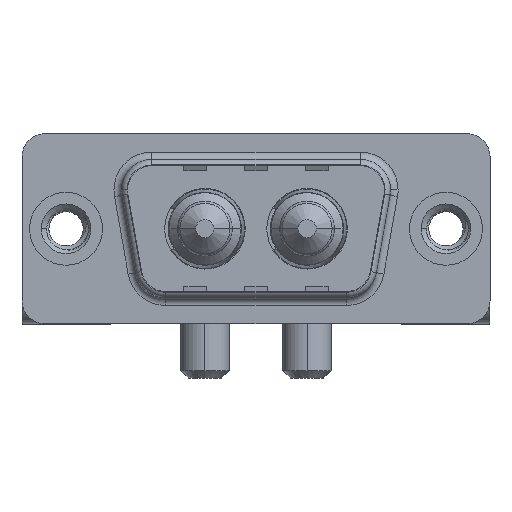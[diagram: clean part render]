
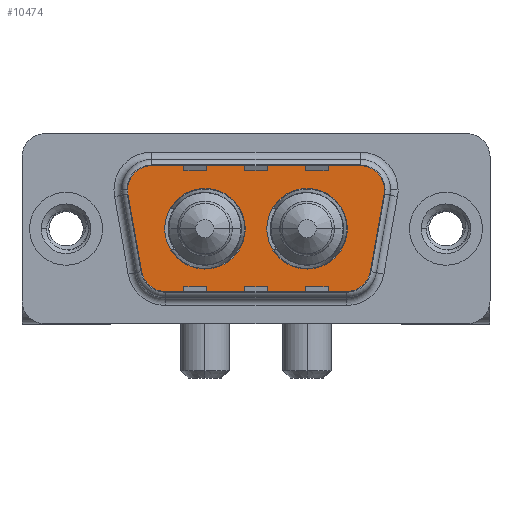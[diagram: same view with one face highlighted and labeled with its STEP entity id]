
A CAD part, top view. The second image highlights one B-rep face of the part: STEP entity #10474.
In plain terms, the highlighted planar face has unit normal (0, 0, 1).
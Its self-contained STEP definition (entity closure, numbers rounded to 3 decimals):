
#266 = CARTESIAN_POINT ( 'NONE',  ( 18.51, 0., 0. ) ) ;
#269 = CARTESIAN_POINT ( 'NONE',  ( 11.79, 0., 0. ) ) ;
#540 = EDGE_CURVE ( 'NONE', #4864, #10879, #11350, .T. ) ;
#550 = DIRECTION ( 'NONE',  ( 1., 0., 0. ) ) ;
#555 = ORIENTED_EDGE ( 'NONE', *, *, #4746, .T. ) ;
#648 = CARTESIAN_POINT ( 'NONE',  ( 5.436, 4.9, 0. ) ) ;
#845 = LINE ( 'NONE', #12289, #9375 ) ;
#884 = CARTESIAN_POINT ( 'NONE',  ( 6.459, -4.9, 0. ) ) ;
#1030 = FACE_OUTER_BOUND ( 'NONE', #4273, .T. ) ;
#1350 = VERTEX_POINT ( 'NONE', #11225 ) ;
#1353 = CARTESIAN_POINT ( 'NONE',  ( 18.541, -4.9, 0. ) ) ;
#1484 = VERTEX_POINT ( 'NONE', #8510 ) ;
#1983 = CARTESIAN_POINT ( 'NONE',  ( 6.459, -4.9, 0. ) ) ;
#2036 = CARTESIAN_POINT ( 'NONE',  ( 9.14, 0., 0. ) ) ;
#2043 = DIRECTION ( 'NONE',  ( 1., 0., 0. ) ) ;
#2102 = CARTESIAN_POINT ( 'NONE',  ( 18.541, -2.9, 0. ) ) ;
#2132 = EDGE_LOOP ( 'NONE', ( #4965, #3068 ) ) ;
#2228 = AXIS2_PLACEMENT_3D ( 'NONE', #5173, #6250, #6369 ) ;
#2273 = VERTEX_POINT ( 'NONE', #12430 ) ;
#2414 = VECTOR ( 'NONE', #12393, 1000. ) ;
#2449 = CARTESIAN_POINT ( 'NONE',  ( 5.436, 2.9, 0. ) ) ;
#2561 = LINE ( 'NONE', #6303, #6663 ) ;
#2609 = EDGE_CURVE ( 'NONE', #2273, #1484, #2561, .T. ) ;
#2627 = DIRECTION ( 'NONE',  ( 0.174, 0.985, 0. ) ) ;
#2643 = DIRECTION ( 'NONE',  ( 1., 0., 0. ) ) ;
#2693 = AXIS2_PLACEMENT_3D ( 'NONE', #9643, #8895, #9904 ) ;
#2695 = EDGE_CURVE ( 'NONE', #10616, #7680, #3641, .T. ) ;
#2728 = LINE ( 'NONE', #884, #2414 ) ;
#2748 = CARTESIAN_POINT ( 'NONE',  ( 15.86, 0., 0. ) ) ;
#2749 = VERTEX_POINT ( 'NONE', #269 ) ;
#2853 = AXIS2_PLACEMENT_3D ( 'NONE', #8465, #7459, #2643 ) ;
#2982 = ORIENTED_EDGE ( 'NONE', *, *, #3507, .F. ) ;
#2987 = DIRECTION ( 'NONE',  ( 0., 0., 1. ) ) ;
#3068 = ORIENTED_EDGE ( 'NONE', *, *, #9270, .F. ) ;
#3157 = AXIS2_PLACEMENT_3D ( 'NONE', #3383, #8386, #9260 ) ;
#3383 = CARTESIAN_POINT ( 'NONE',  ( 9.14, 0., 0. ) ) ;
#3507 = EDGE_CURVE ( 'NONE', #7680, #10616, #8321, .T. ) ;
#3641 = CIRCLE ( 'NONE', #8900, 2.65 ) ;
#3731 = CARTESIAN_POINT ( 'NONE',  ( 3.466, 2.553, 0. ) ) ;
#4209 = ORIENTED_EDGE ( 'NONE', *, *, #4969, .T. ) ;
#4273 = EDGE_LOOP ( 'NONE', ( #555, #5560, #10029, #4429, #10700, #5777, #8716, #11575, #4209 ) ) ;
#4429 = ORIENTED_EDGE ( 'NONE', *, *, #5820, .T. ) ;
#4691 = EDGE_CURVE ( 'NONE', #1484, #1350, #5625, .T. ) ;
#4746 = EDGE_CURVE ( 'NONE', #7253, #2273, #5834, .T. ) ;
#4842 = CARTESIAN_POINT ( 'NONE',  ( 6.49, 0., 0. ) ) ;
#4851 = EDGE_LOOP ( 'NONE', ( #5051, #2982 ) ) ;
#4864 = VERTEX_POINT ( 'NONE', #648 ) ;
#4965 = ORIENTED_EDGE ( 'NONE', *, *, #6888, .F. ) ;
#4969 = EDGE_CURVE ( 'NONE', #12478, #7253, #2728, .T. ) ;
#5015 = DIRECTION ( 'NONE',  ( -1., 0., 0. ) ) ;
#5051 = ORIENTED_EDGE ( 'NONE', *, *, #2695, .F. ) ;
#5173 = CARTESIAN_POINT ( 'NONE',  ( 19.564, 2.9, 0. ) ) ;
#5437 = AXIS2_PLACEMENT_3D ( 'NONE', #2102, #11718, #9818 ) ;
#5560 = ORIENTED_EDGE ( 'NONE', *, *, #2609, .T. ) ;
#5625 = CIRCLE ( 'NONE', #8866, 2. ) ;
#5742 = AXIS2_PLACEMENT_3D ( 'NONE', #7564, #2987, #2043 ) ;
#5777 = ORIENTED_EDGE ( 'NONE', *, *, #540, .T. ) ;
#5820 = EDGE_CURVE ( 'NONE', #1350, #9046, #8099, .T. ) ;
#5834 = CIRCLE ( 'NONE', #5437, 2. ) ;
#5887 = CARTESIAN_POINT ( 'NONE',  ( 5.436, 4.9, 0. ) ) ;
#6202 = VERTEX_POINT ( 'NONE', #10656 ) ;
#6218 = VERTEX_POINT ( 'NONE', #4842 ) ;
#6250 = DIRECTION ( 'NONE',  ( 0., 0., 1. ) ) ;
#6303 = CARTESIAN_POINT ( 'NONE',  ( 21.534, 2.553, 0. ) ) ;
#6369 = DIRECTION ( 'NONE',  ( -1., 0., 0. ) ) ;
#6539 = DIRECTION ( 'NONE',  ( 0., 0., 1. ) ) ;
#6663 = VECTOR ( 'NONE', #2627, 1000. ) ;
#6888 = EDGE_CURVE ( 'NONE', #2749, #6218, #10901, .T. ) ;
#6980 = DIRECTION ( 'NONE',  ( 0., 0., 1. ) ) ;
#7253 = VERTEX_POINT ( 'NONE', #1353 ) ;
#7459 = DIRECTION ( 'NONE',  ( 0., 0., 1. ) ) ;
#7564 = CARTESIAN_POINT ( 'NONE',  ( 18.541, -2.9, 0. ) ) ;
#7680 = VERTEX_POINT ( 'NONE', #10129 ) ;
#7810 = FACE_BOUND ( 'NONE', #2132, .T. ) ;
#7817 = CIRCLE ( 'NONE', #3157, 2.65 ) ;
#7994 = CARTESIAN_POINT ( 'NONE',  ( 19.564, 2.9, 0. ) ) ;
#8099 = CIRCLE ( 'NONE', #2228, 2. ) ;
#8321 = CIRCLE ( 'NONE', #2853, 2.65 ) ;
#8386 = DIRECTION ( 'NONE',  ( 0., 0., 1. ) ) ;
#8465 = CARTESIAN_POINT ( 'NONE',  ( 15.86, 0., 0. ) ) ;
#8510 = CARTESIAN_POINT ( 'NONE',  ( 21.534, 2.553, 0. ) ) ;
#8563 = DIRECTION ( 'NONE',  ( 0., 0., 1. ) ) ;
#8716 = ORIENTED_EDGE ( 'NONE', *, *, #12156, .T. ) ;
#8738 = LINE ( 'NONE', #5887, #8808 ) ;
#8802 = DIRECTION ( 'NONE',  ( 0.174, -0.985, 0. ) ) ;
#8808 = VECTOR ( 'NONE', #11516, 1000. ) ;
#8863 = EDGE_CURVE ( 'NONE', #9046, #4864, #8738, .T. ) ;
#8866 = AXIS2_PLACEMENT_3D ( 'NONE', #7994, #6980, #5015 ) ;
#8895 = DIRECTION ( 'NONE',  ( 0., 0., 1. ) ) ;
#8900 = AXIS2_PLACEMENT_3D ( 'NONE', #2748, #6539, #12411 ) ;
#9046 = VERTEX_POINT ( 'NONE', #11736 ) ;
#9215 = DIRECTION ( 'NONE',  ( 0., 0., 1. ) ) ;
#9260 = DIRECTION ( 'NONE',  ( 1., 0., 0. ) ) ;
#9270 = EDGE_CURVE ( 'NONE', #6218, #2749, #7817, .T. ) ;
#9369 = CIRCLE ( 'NONE', #2693, 2. ) ;
#9375 = VECTOR ( 'NONE', #8802, 1000. ) ;
#9643 = CARTESIAN_POINT ( 'NONE',  ( 6.459, -2.9, 0. ) ) ;
#9693 = FACE_BOUND ( 'NONE', #4851, .T. ) ;
#9751 = DIRECTION ( 'NONE',  ( 1., 0., 0. ) ) ;
#9818 = DIRECTION ( 'NONE',  ( 1., 0., 0. ) ) ;
#9904 = DIRECTION ( 'NONE',  ( -1., 0., 0. ) ) ;
#10029 = ORIENTED_EDGE ( 'NONE', *, *, #4691, .T. ) ;
#10129 = CARTESIAN_POINT ( 'NONE',  ( 13.21, 0., 0. ) ) ;
#10474 = ADVANCED_FACE ( 'NONE', ( #9693, #7810, #1030 ), #11657, .T. ) ;
#10517 = AXIS2_PLACEMENT_3D ( 'NONE', #2449, #9215, #550 ) ;
#10616 = VERTEX_POINT ( 'NONE', #266 ) ;
#10656 = CARTESIAN_POINT ( 'NONE',  ( 4.489, -3.247, 0. ) ) ;
#10700 = ORIENTED_EDGE ( 'NONE', *, *, #8863, .T. ) ;
#10879 = VERTEX_POINT ( 'NONE', #3731 ) ;
#10901 = CIRCLE ( 'NONE', #11912, 2.65 ) ;
#11225 = CARTESIAN_POINT ( 'NONE',  ( 21.564, 2.9, 0. ) ) ;
#11350 = CIRCLE ( 'NONE', #10517, 2. ) ;
#11516 = DIRECTION ( 'NONE',  ( -1., 0., 0. ) ) ;
#11575 = ORIENTED_EDGE ( 'NONE', *, *, #11903, .T. ) ;
#11657 = PLANE ( 'NONE',  #5742 ) ;
#11718 = DIRECTION ( 'NONE',  ( 0., 0., 1. ) ) ;
#11736 = CARTESIAN_POINT ( 'NONE',  ( 19.564, 4.9, 0. ) ) ;
#11903 = EDGE_CURVE ( 'NONE', #6202, #12478, #9369, .T. ) ;
#11912 = AXIS2_PLACEMENT_3D ( 'NONE', #2036, #8563, #9751 ) ;
#12156 = EDGE_CURVE ( 'NONE', #10879, #6202, #845, .T. ) ;
#12289 = CARTESIAN_POINT ( 'NONE',  ( 3.466, 2.553, 0. ) ) ;
#12393 = DIRECTION ( 'NONE',  ( 1., 0., 0. ) ) ;
#12411 = DIRECTION ( 'NONE',  ( 1., 0., 0. ) ) ;
#12430 = CARTESIAN_POINT ( 'NONE',  ( 20.511, -3.247, 0. ) ) ;
#12478 = VERTEX_POINT ( 'NONE', #1983 ) ;
